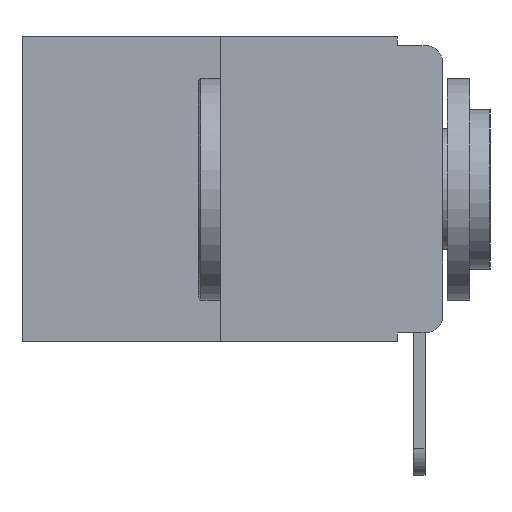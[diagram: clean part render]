
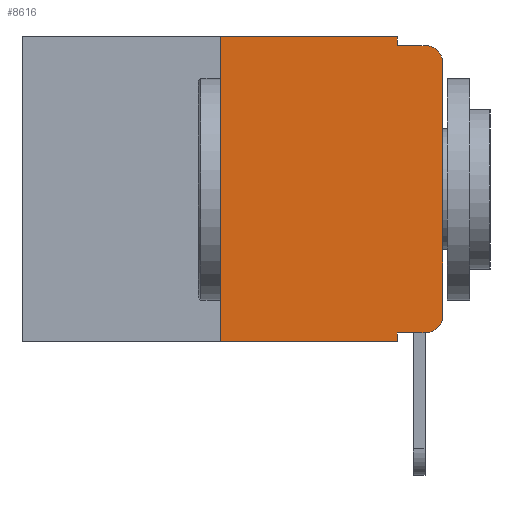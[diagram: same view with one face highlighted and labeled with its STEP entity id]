
A CAD part, left-side view. The second image highlights one B-rep face of the part: STEP entity #8616.
In plain terms, the highlighted planar face has unit normal (-1, 0, 0).
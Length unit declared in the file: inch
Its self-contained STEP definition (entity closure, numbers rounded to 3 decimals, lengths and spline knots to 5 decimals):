
#28 = ORIENTED_EDGE ( 'NONE', *, *, #14716, .F. ) ;
#48 = ORIENTED_EDGE ( 'NONE', *, *, #8158, .T. ) ;
#507 = EDGE_CURVE ( 'NONE', #12959, #11717, #16780, .T. ) ;
#631 = ORIENTED_EDGE ( 'NONE', *, *, #20834, .F. ) ;
#789 = CARTESIAN_POINT ( 'NONE',  ( 0., 0.051, 0. ) ) ;
#1141 = LINE ( 'NONE', #21088, #6053 ) ;
#1970 = VECTOR ( 'NONE', #7762, 39.37008 ) ;
#2410 = VERTEX_POINT ( 'NONE', #18452 ) ;
#2711 = VECTOR ( 'NONE', #17837, 39.37008 ) ;
#3631 = CARTESIAN_POINT ( 'NONE',  ( 0., 0.02, -0.313 ) ) ;
#4425 = CARTESIAN_POINT ( 'NONE',  ( 0., 0.051, -0.01 ) ) ;
#4878 = EDGE_CURVE ( 'NONE', #14307, #11717, #1141, .T. ) ;
#4900 = AXIS2_PLACEMENT_3D ( 'NONE', #13865, #10077, #6304 ) ;
#5212 = LINE ( 'NONE', #7947, #2711 ) ;
#5349 = VERTEX_POINT ( 'NONE', #21877 ) ;
#5398 = CARTESIAN_POINT ( 'NONE',  ( 0., 0., 0. ) ) ;
#6053 = VECTOR ( 'NONE', #15458, 39.37008 ) ;
#6304 = DIRECTION ( 'NONE',  ( 0., 0., -1. ) ) ;
#6693 = VERTEX_POINT ( 'NONE', #15683 ) ;
#7110 = CARTESIAN_POINT ( 'NONE',  ( 0., 0.02, -0.333 ) ) ;
#7762 = DIRECTION ( 'NONE',  ( 0., -1., 0. ) ) ;
#7947 = CARTESIAN_POINT ( 'NONE',  ( 0., 0.051, -0.333 ) ) ;
#8158 = EDGE_CURVE ( 'NONE', #12959, #14409, #5212, .T. ) ;
#8616 = ADVANCED_FACE ( 'NONE', ( #10970 ), #20499, .F. ) ;
#9048 = CARTESIAN_POINT ( 'NONE',  ( 0., 0.051, -0.343 ) ) ;
#9380 = EDGE_CURVE ( 'NONE', #5349, #18850, #23556, .T. ) ;
#9559 = DIRECTION ( 'NONE',  ( 0., -1., 0. ) ) ;
#10077 = DIRECTION ( 'NONE',  ( -1., 0., 0. ) ) ;
#10592 = CARTESIAN_POINT ( 'NONE',  ( 0., 0.473, 0. ) ) ;
#10689 = ORIENTED_EDGE ( 'NONE', *, *, #18671, .F. ) ;
#10970 = FACE_OUTER_BOUND ( 'NONE', #19512, .T. ) ;
#11109 = CARTESIAN_POINT ( 'NONE',  ( 0., 0.051, -0.333 ) ) ;
#11601 = CARTESIAN_POINT ( 'NONE',  ( 0., 0.051, -0.01 ) ) ;
#11713 = VECTOR ( 'NONE', #17392, 39.37008 ) ;
#11717 = VERTEX_POINT ( 'NONE', #9048 ) ;
#11875 = CARTESIAN_POINT ( 'NONE',  ( 0., 0.051, 0. ) ) ;
#12219 = CARTESIAN_POINT ( 'NONE',  ( 0., 0.25, -0.343 ) ) ;
#12445 = ORIENTED_EDGE ( 'NONE', *, *, #16055, .F. ) ;
#12701 = CARTESIAN_POINT ( 'NONE',  ( 0., 0., -0.03 ) ) ;
#12959 = VERTEX_POINT ( 'NONE', #11109 ) ;
#13027 = LINE ( 'NONE', #11601, #1970 ) ;
#13252 = DIRECTION ( 'NONE',  ( 0., 0., 1. ) ) ;
#13400 = CARTESIAN_POINT ( 'NONE',  ( 0., 0.25, 0. ) ) ;
#13865 = CARTESIAN_POINT ( 'NONE',  ( 0., 0.02, -0.03 ) ) ;
#14066 = VERTEX_POINT ( 'NONE', #4425 ) ;
#14307 = VERTEX_POINT ( 'NONE', #12219 ) ;
#14409 = VERTEX_POINT ( 'NONE', #7110 ) ;
#14716 = EDGE_CURVE ( 'NONE', #6693, #23610, #15247, .T. ) ;
#15176 = VECTOR ( 'NONE', #23123, 39.37008 ) ;
#15247 = LINE ( 'NONE', #25097, #22968 ) ;
#15287 = ORIENTED_EDGE ( 'NONE', *, *, #9380, .T. ) ;
#15458 = DIRECTION ( 'NONE',  ( 0., -1., 0. ) ) ;
#15683 = CARTESIAN_POINT ( 'NONE',  ( 0., 0.25, 0. ) ) ;
#16055 = EDGE_CURVE ( 'NONE', #23610, #14066, #24085, .T. ) ;
#16412 = CARTESIAN_POINT ( 'NONE',  ( 0., 0.051, 0. ) ) ;
#16780 = LINE ( 'NONE', #16412, #20803 ) ;
#16818 = VECTOR ( 'NONE', #13252, 39.37008 ) ;
#17392 = DIRECTION ( 'NONE',  ( 0., 0., 1. ) ) ;
#17837 = DIRECTION ( 'NONE',  ( 0., -1., 0. ) ) ;
#18145 = ORIENTED_EDGE ( 'NONE', *, *, #507, .F. ) ;
#18231 = ORIENTED_EDGE ( 'NONE', *, *, #4878, .T. ) ;
#18452 = CARTESIAN_POINT ( 'NONE',  ( 0., 0.02, -0.01 ) ) ;
#18525 = DIRECTION ( 'NONE',  ( 0., 0., -1. ) ) ;
#18671 = EDGE_CURVE ( 'NONE', #14066, #2410, #13027, .T. ) ;
#18848 = CIRCLE ( 'NONE', #4900, 0.02 ) ;
#18850 = VERTEX_POINT ( 'NONE', #12701 ) ;
#19050 = ORIENTED_EDGE ( 'NONE', *, *, #19970, .T. ) ;
#19171 = EDGE_CURVE ( 'NONE', #14409, #5349, #22592, .T. ) ;
#19512 = EDGE_LOOP ( 'NONE', ( #15287, #19050, #10689, #12445, #28, #631, #18231, #18145, #48, #21586 ) ) ;
#19537 = DIRECTION ( 'NONE',  ( 0., 0., -1. ) ) ;
#19970 = EDGE_CURVE ( 'NONE', #18850, #2410, #18848, .T. ) ;
#20237 = DIRECTION ( 'NONE',  ( 1., 0., 0. ) ) ;
#20386 = DIRECTION ( 'NONE',  ( 0., 0., -1. ) ) ;
#20499 = PLANE ( 'NONE',  #24828 ) ;
#20803 = VECTOR ( 'NONE', #20386, 39.37008 ) ;
#20834 = EDGE_CURVE ( 'NONE', #14307, #6693, #24361, .T. ) ;
#21088 = CARTESIAN_POINT ( 'NONE',  ( 0., 0.473, -0.343 ) ) ;
#21586 = ORIENTED_EDGE ( 'NONE', *, *, #19171, .T. ) ;
#21877 = CARTESIAN_POINT ( 'NONE',  ( 0., 0., -0.313 ) ) ;
#22592 = CIRCLE ( 'NONE', #23800, 0.02 ) ;
#22968 = VECTOR ( 'NONE', #9559, 39.37008 ) ;
#23123 = DIRECTION ( 'NONE',  ( 0., 0., -1. ) ) ;
#23392 = DIRECTION ( 'NONE',  ( -1., 0., 0. ) ) ;
#23556 = LINE ( 'NONE', #5398, #16818 ) ;
#23610 = VERTEX_POINT ( 'NONE', #789 ) ;
#23800 = AXIS2_PLACEMENT_3D ( 'NONE', #3631, #23392, #19537 ) ;
#24085 = LINE ( 'NONE', #11875, #15176 ) ;
#24361 = LINE ( 'NONE', #13400, #11713 ) ;
#24828 = AXIS2_PLACEMENT_3D ( 'NONE', #10592, #20237, #18525 ) ;
#25097 = CARTESIAN_POINT ( 'NONE',  ( 0., 0.473, 0. ) ) ;
